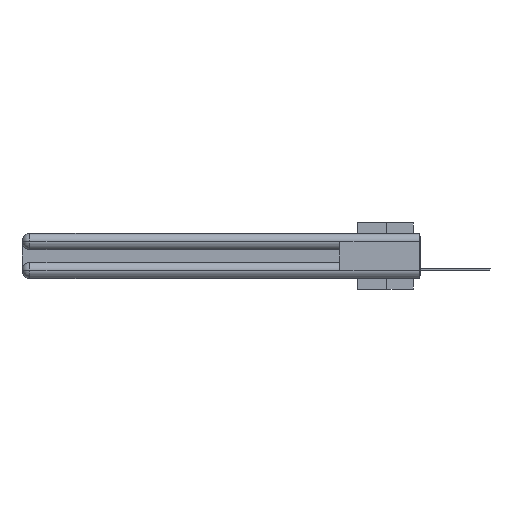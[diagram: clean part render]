
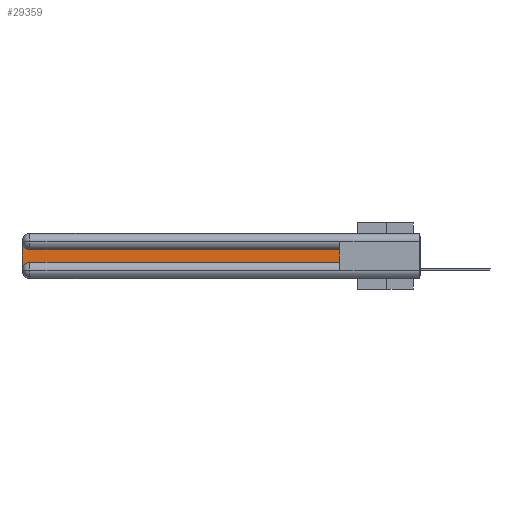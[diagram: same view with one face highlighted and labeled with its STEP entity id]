
A CAD part, left-side view. The second image highlights one B-rep face of the part: STEP entity #29359.
In plain terms, the highlighted planar face has unit normal (-1, 0, 0).
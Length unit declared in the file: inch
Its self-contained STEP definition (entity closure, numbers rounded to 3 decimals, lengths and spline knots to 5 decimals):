
#3261 = EDGE_CURVE ( 'NONE', #5352, #5424, #7746, .T. ) ;
#4054 = PLANE ( 'NONE',  #21863 ) ;
#4261 = VERTEX_POINT ( 'NONE', #17123 ) ;
#4902 = CARTESIAN_POINT ( 'NONE',  ( 0.075, 2.94, -0.0625 ) ) ;
#5140 = DIRECTION ( 'NONE',  ( 1., 0., 0. ) ) ;
#5352 = VERTEX_POINT ( 'NONE', #17431 ) ;
#5424 = VERTEX_POINT ( 'NONE', #12476 ) ;
#5627 = DIRECTION ( 'NONE',  ( 0., 0., 1. ) ) ;
#7746 = LINE ( 'NONE', #36147, #22200 ) ;
#8872 = ORIENTED_EDGE ( 'NONE', *, *, #10267, .T. ) ;
#9813 = DIRECTION ( 'NONE',  ( 0., 0., -1. ) ) ;
#10267 = EDGE_CURVE ( 'NONE', #4261, #28847, #26074, .T. ) ;
#11966 = CARTESIAN_POINT ( 'NONE',  ( 0.075, 3., -0.0625 ) ) ;
#12476 = CARTESIAN_POINT ( 'NONE',  ( 0.075, 2.94, -0.1225 ) ) ;
#12621 = EDGE_LOOP ( 'NONE', ( #20356, #27121, #21450, #25696, #8872, #24314 ) ) ;
#12750 = CARTESIAN_POINT ( 'NONE',  ( 0.075, 3., -0.1225 ) ) ;
#13794 = AXIS2_PLACEMENT_3D ( 'NONE', #30430, #22056, #25263 ) ;
#14270 = VECTOR ( 'NONE', #5627, 39.37008 ) ;
#15113 = AXIS2_PLACEMENT_3D ( 'NONE', #4902, #5140, #33142 ) ;
#15945 = VECTOR ( 'NONE', #24377, 39.37008 ) ;
#16343 = CARTESIAN_POINT ( 'NONE',  ( 0.075, 0.6, -0.2175 ) ) ;
#16443 = CARTESIAN_POINT ( 'NONE',  ( 0.075, 0.6, -0.2175 ) ) ;
#17123 = CARTESIAN_POINT ( 'NONE',  ( 0.075, 2.94, -0.2175 ) ) ;
#17431 = CARTESIAN_POINT ( 'NONE',  ( 0.075, 0.6, -0.1225 ) ) ;
#19370 = EDGE_CURVE ( 'NONE', #20430, #4261, #32059, .T. ) ;
#19848 = VECTOR ( 'NONE', #26680, 39.37008 ) ;
#20356 = ORIENTED_EDGE ( 'NONE', *, *, #3261, .T. ) ;
#20430 = VERTEX_POINT ( 'NONE', #33637 ) ;
#21450 = ORIENTED_EDGE ( 'NONE', *, *, #28022, .T. ) ;
#21863 = AXIS2_PLACEMENT_3D ( 'NONE', #12750, #23445, #9813 ) ;
#21940 = CARTESIAN_POINT ( 'NONE',  ( 0.075, 0.6, -0.2175 ) ) ;
#22056 = DIRECTION ( 'NONE',  ( 1., 0., 0. ) ) ;
#22200 = VECTOR ( 'NONE', #24973, 39.37008 ) ;
#23445 = DIRECTION ( 'NONE',  ( 1., 0., 0. ) ) ;
#24314 = ORIENTED_EDGE ( 'NONE', *, *, #33465, .T. ) ;
#24377 = DIRECTION ( 'NONE',  ( 0., -1., 0. ) ) ;
#24778 = VERTEX_POINT ( 'NONE', #11966 ) ;
#24973 = DIRECTION ( 'NONE',  ( 0., 1., 0. ) ) ;
#25263 = DIRECTION ( 'NONE',  ( 0., 0., -1. ) ) ;
#25329 = LINE ( 'NONE', #21940, #14270 ) ;
#25696 = ORIENTED_EDGE ( 'NONE', *, *, #19370, .T. ) ;
#26074 = LINE ( 'NONE', #16443, #15945 ) ;
#26680 = DIRECTION ( 'NONE',  ( 0., 0., -1. ) ) ;
#27121 = ORIENTED_EDGE ( 'NONE', *, *, #30623, .T. ) ;
#27414 = LINE ( 'NONE', #32341, #19848 ) ;
#28022 = EDGE_CURVE ( 'NONE', #24778, #20430, #27414, .T. ) ;
#28847 = VERTEX_POINT ( 'NONE', #16343 ) ;
#29359 = ADVANCED_FACE ( 'NONE', ( #35678 ), #4054, .F. ) ;
#30430 = CARTESIAN_POINT ( 'NONE',  ( 0.075, 2.94, -0.2775 ) ) ;
#30623 = EDGE_CURVE ( 'NONE', #5424, #24778, #33490, .T. ) ;
#32059 = CIRCLE ( 'NONE', #13794, 0.06 ) ;
#32341 = CARTESIAN_POINT ( 'NONE',  ( 0.075, 3., -0.2175 ) ) ;
#33142 = DIRECTION ( 'NONE',  ( 0., 0., -1. ) ) ;
#33465 = EDGE_CURVE ( 'NONE', #28847, #5352, #25329, .T. ) ;
#33490 = CIRCLE ( 'NONE', #15113, 0.06 ) ;
#33637 = CARTESIAN_POINT ( 'NONE',  ( 0.075, 3., -0.2775 ) ) ;
#35678 = FACE_OUTER_BOUND ( 'NONE', #12621, .T. ) ;
#36147 = CARTESIAN_POINT ( 'NONE',  ( 0.075, 0.6, -0.1225 ) ) ;
